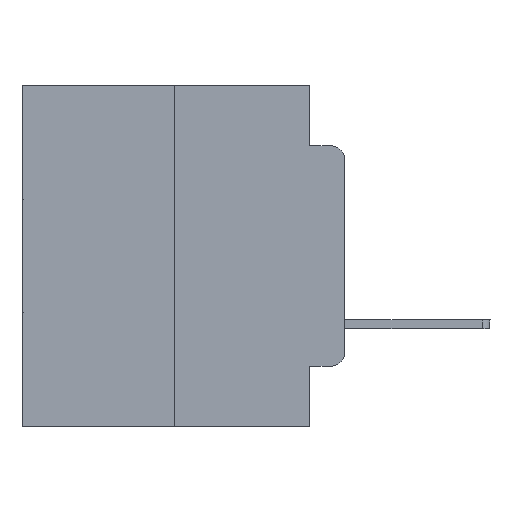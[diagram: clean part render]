
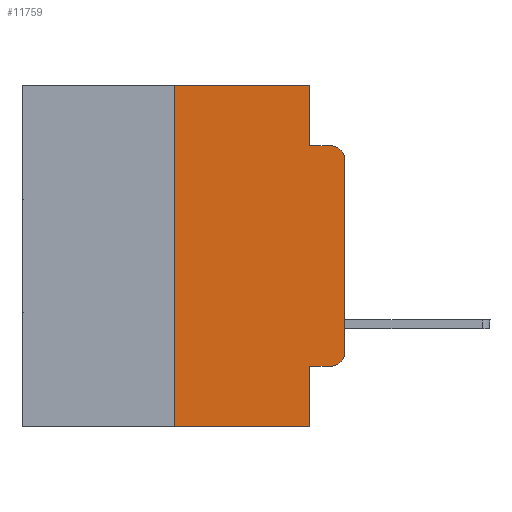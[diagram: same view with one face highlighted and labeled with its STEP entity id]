
A CAD part, left-side view. The second image highlights one B-rep face of the part: STEP entity #11759.
In plain terms, the highlighted planar face has unit normal (-1, 0, 0).
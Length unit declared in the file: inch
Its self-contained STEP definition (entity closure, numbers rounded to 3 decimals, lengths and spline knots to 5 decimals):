
#178 = DIRECTION ( 'NONE',  ( 0., 0., -1. ) ) ;
#320 = ORIENTED_EDGE ( 'NONE', *, *, #20053, .F. ) ;
#361 = EDGE_CURVE ( 'NONE', #21486, #19622, #7211, .T. ) ;
#375 = CARTESIAN_POINT ( 'NONE',  ( 0., 0.02, -0.4115 ) ) ;
#494 = CARTESIAN_POINT ( 'NONE',  ( 0., 0.25, 0. ) ) ;
#539 = CARTESIAN_POINT ( 'NONE',  ( 0., 0.051, 0. ) ) ;
#771 = LINE ( 'NONE', #494, #19558 ) ;
#1230 = LINE ( 'NONE', #22197, #9539 ) ;
#1393 = DIRECTION ( 'NONE',  ( -1., 0., 0. ) ) ;
#2260 = FACE_OUTER_BOUND ( 'NONE', #27531, .T. ) ;
#2411 = LINE ( 'NONE', #15263, #9622 ) ;
#2510 = ORIENTED_EDGE ( 'NONE', *, *, #17015, .T. ) ;
#2735 = CIRCLE ( 'NONE', #10332, 0.02 ) ;
#2785 = EDGE_CURVE ( 'NONE', #22533, #19622, #2735, .T. ) ;
#4343 = EDGE_CURVE ( 'NONE', #25978, #25469, #7428, .T. ) ;
#5122 = AXIS2_PLACEMENT_3D ( 'NONE', #5657, #5927, #18482 ) ;
#5123 = VECTOR ( 'NONE', #18452, 39.37008 ) ;
#5606 = EDGE_CURVE ( 'NONE', #5973, #22533, #21840, .T. ) ;
#5657 = CARTESIAN_POINT ( 'NONE',  ( 0., 0.02, -0.3915 ) ) ;
#5927 = DIRECTION ( 'NONE',  ( -1., 0., 0. ) ) ;
#5973 = VERTEX_POINT ( 'NONE', #19422 ) ;
#7211 = LINE ( 'NONE', #11673, #7258 ) ;
#7258 = VECTOR ( 'NONE', #15704, 39.37008 ) ;
#7428 = LINE ( 'NONE', #24163, #14808 ) ;
#7540 = DIRECTION ( 'NONE',  ( 0., -1., 0. ) ) ;
#7588 = CARTESIAN_POINT ( 'NONE',  ( 0., 0.051, -0.0885 ) ) ;
#8899 = EDGE_CURVE ( 'NONE', #12893, #11500, #20553, .T. ) ;
#9539 = VECTOR ( 'NONE', #7540, 39.37008 ) ;
#9622 = VECTOR ( 'NONE', #17075, 39.37008 ) ;
#9830 = CARTESIAN_POINT ( 'NONE',  ( 0., 0.25, 0. ) ) ;
#9960 = CARTESIAN_POINT ( 'NONE',  ( 0., 0.051, -0.4115 ) ) ;
#10332 = AXIS2_PLACEMENT_3D ( 'NONE', #24593, #1393, #16207 ) ;
#10648 = ORIENTED_EDGE ( 'NONE', *, *, #4343, .F. ) ;
#10740 = ORIENTED_EDGE ( 'NONE', *, *, #24173, .F. ) ;
#10800 = PLANE ( 'NONE',  #13374 ) ;
#10962 = CARTESIAN_POINT ( 'NONE',  ( 0., 0., 0. ) ) ;
#11270 = CARTESIAN_POINT ( 'NONE',  ( 0., 0.051, 0. ) ) ;
#11309 = DIRECTION ( 'NONE',  ( 0., 0., -1. ) ) ;
#11500 = VERTEX_POINT ( 'NONE', #375 ) ;
#11673 = CARTESIAN_POINT ( 'NONE',  ( 0., 0.051, -0.0885 ) ) ;
#11678 = DIRECTION ( 'NONE',  ( 0., 0., 1. ) ) ;
#11759 = ADVANCED_FACE ( 'NONE', ( #2260 ), #10800, .F. ) ;
#12893 = VERTEX_POINT ( 'NONE', #16006 ) ;
#13112 = ORIENTED_EDGE ( 'NONE', *, *, #5606, .T. ) ;
#13374 = AXIS2_PLACEMENT_3D ( 'NONE', #21557, #19036, #178 ) ;
#14808 = VECTOR ( 'NONE', #20263, 39.37008 ) ;
#15263 = CARTESIAN_POINT ( 'NONE',  ( 0., 0.051, 0. ) ) ;
#15704 = DIRECTION ( 'NONE',  ( 0., -1., 0. ) ) ;
#15738 = VECTOR ( 'NONE', #17764, 39.37008 ) ;
#15931 = ORIENTED_EDGE ( 'NONE', *, *, #361, .F. ) ;
#16006 = CARTESIAN_POINT ( 'NONE',  ( 0., 0.051, -0.4115 ) ) ;
#16207 = DIRECTION ( 'NONE',  ( 0., 0., -1. ) ) ;
#16630 = CARTESIAN_POINT ( 'NONE',  ( 0., 0.25, -0.5 ) ) ;
#16999 = ORIENTED_EDGE ( 'NONE', *, *, #8899, .T. ) ;
#17015 = EDGE_CURVE ( 'NONE', #20257, #19237, #1230, .T. ) ;
#17075 = DIRECTION ( 'NONE',  ( 0., 0., -1. ) ) ;
#17297 = LINE ( 'NONE', #539, #24948 ) ;
#17523 = CARTESIAN_POINT ( 'NONE',  ( 0., 0.02, -0.0885 ) ) ;
#17554 = CARTESIAN_POINT ( 'NONE',  ( 0., 0.051, -0.5 ) ) ;
#17764 = DIRECTION ( 'NONE',  ( 0., 0., 1. ) ) ;
#18063 = EDGE_CURVE ( 'NONE', #11500, #5973, #20301, .T. ) ;
#18452 = DIRECTION ( 'NONE',  ( 0., -1., 0. ) ) ;
#18482 = DIRECTION ( 'NONE',  ( 0., 0., -1. ) ) ;
#19036 = DIRECTION ( 'NONE',  ( 1., 0., 0. ) ) ;
#19098 = ORIENTED_EDGE ( 'NONE', *, *, #24878, .F. ) ;
#19237 = VERTEX_POINT ( 'NONE', #17554 ) ;
#19422 = CARTESIAN_POINT ( 'NONE',  ( 0., 0., -0.3915 ) ) ;
#19558 = VECTOR ( 'NONE', #11678, 39.37008 ) ;
#19622 = VERTEX_POINT ( 'NONE', #17523 ) ;
#20053 = EDGE_CURVE ( 'NONE', #25469, #21486, #2411, .T. ) ;
#20230 = ORIENTED_EDGE ( 'NONE', *, *, #2785, .T. ) ;
#20257 = VERTEX_POINT ( 'NONE', #16630 ) ;
#20263 = DIRECTION ( 'NONE',  ( 0., -1., 0. ) ) ;
#20301 = CIRCLE ( 'NONE', #5122, 0.02 ) ;
#20553 = LINE ( 'NONE', #9960, #5123 ) ;
#21486 = VERTEX_POINT ( 'NONE', #7588 ) ;
#21557 = CARTESIAN_POINT ( 'NONE',  ( 0., 0.473, 0. ) ) ;
#21840 = LINE ( 'NONE', #10962, #15738 ) ;
#22197 = CARTESIAN_POINT ( 'NONE',  ( 0., 0.473, -0.5 ) ) ;
#22533 = VERTEX_POINT ( 'NONE', #27045 ) ;
#24163 = CARTESIAN_POINT ( 'NONE',  ( 0., 0.473, 0. ) ) ;
#24173 = EDGE_CURVE ( 'NONE', #20257, #25978, #771, .T. ) ;
#24332 = ORIENTED_EDGE ( 'NONE', *, *, #18063, .T. ) ;
#24593 = CARTESIAN_POINT ( 'NONE',  ( 0., 0.02, -0.1085 ) ) ;
#24878 = EDGE_CURVE ( 'NONE', #12893, #19237, #17297, .T. ) ;
#24948 = VECTOR ( 'NONE', #11309, 39.37008 ) ;
#25469 = VERTEX_POINT ( 'NONE', #11270 ) ;
#25978 = VERTEX_POINT ( 'NONE', #9830 ) ;
#27045 = CARTESIAN_POINT ( 'NONE',  ( 0., 0., -0.1085 ) ) ;
#27531 = EDGE_LOOP ( 'NONE', ( #13112, #20230, #15931, #320, #10648, #10740, #2510, #19098, #16999, #24332 ) ) ;
